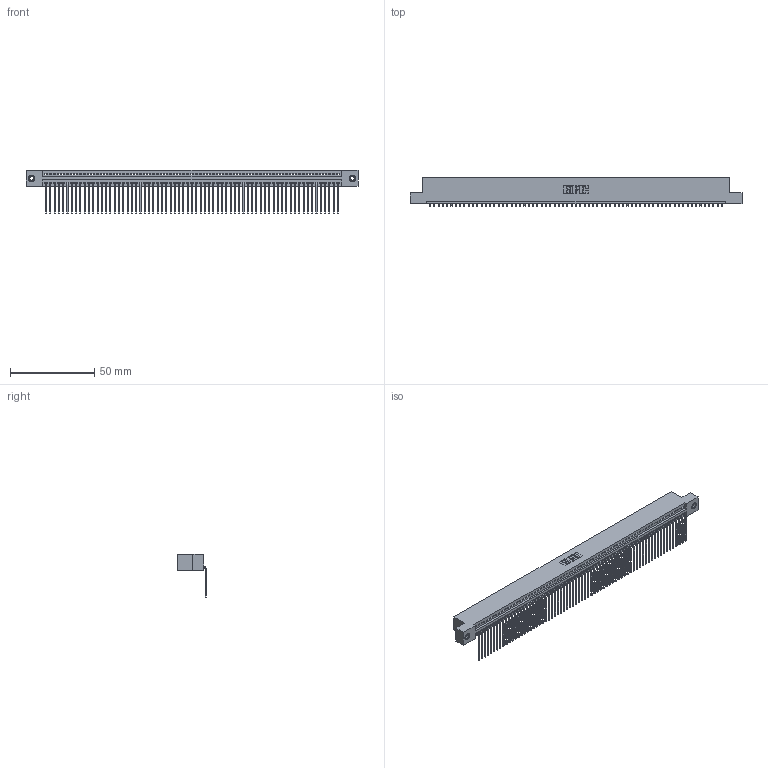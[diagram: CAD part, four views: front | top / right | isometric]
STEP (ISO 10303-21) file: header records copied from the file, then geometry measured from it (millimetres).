
FILE_DESCRIPTION (( 'STEP AP203' ), '1' );
FILE_NAME ('345-069-559-108.STEP', '2019-10-12T13:28:22', ( '' ), ( '' ), 'SwSTEP 2.0', 'SolidWorks 2016', '' );
FILE_SCHEMA (( 'CONFIG_CONTROL_DESIGN' ));
Length unit declared in the file: inch
Products named in the file (4): 345-292-001_558 559 Tail - 1; 345-069-559-108; 345-250-001_345-250-003-102; 345 Part_Flush Mounting Lugs - 0.156 Dia-TI
Assembly tree (72 placements, depth 2):
  345-069-559-108
    345 Part_Flush Mounting Lugs - 0.156 Dia-TI
    345-292-001_558 559 Tail - 1  x69
    345-250-001_345-250-003-102  x2
Bounding box: 196.47 x 16.75 x 25.53 mm (x, y, z)
Volume: 19105.4 mm3; surface area: 27126.3 mm2
Topology: 72 solids, 72 shells, 4326 faces, 13035 edges, 8590 vertices
Faces by surface type: plane 3010, cylinder 1300, cone 12, torus 4
Entity records: 49566 total; most frequent: CARTESIAN_POINT 8566, ORIENTED_EDGE 8562, DIRECTION 7469, EDGE_CURVE 4281, LINE 3853, VECTOR 3853, VERTEX_POINT 2848, AXIS2_PLACEMENT_3D 1808
